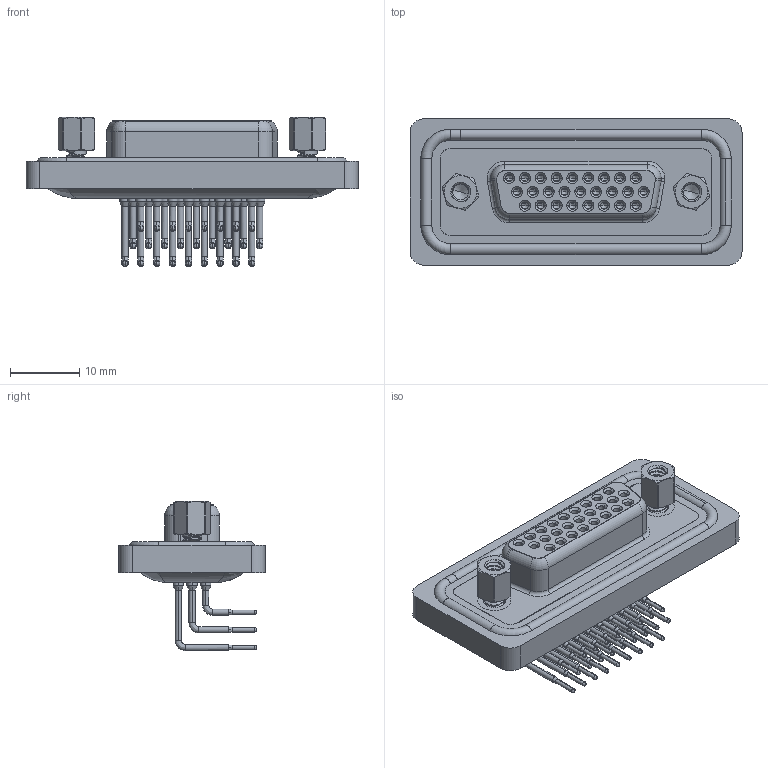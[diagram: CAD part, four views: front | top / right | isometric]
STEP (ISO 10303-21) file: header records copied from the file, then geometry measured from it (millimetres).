
FILE_DESCRIPTION (( 'STEP AP203' ), '1' );
FILE_NAME ('634-W26-662-012.STEP', '2024-04-12T19:19:04', ( '' ), ( '' ), 'SwSTEP 2.0', 'SolidWorks 2023', '' );
FILE_SCHEMA (( 'CONFIG_CONTROL_DESIGN' ));
Length unit declared in the file: millimetre
Products named in the file (9): 634-W26-662-012; 634W 4-40 Hex Standoff; 634W Contact Row 1; 634W Contact Row 2; 634W 4-40 Threaded Rivet; 634W Waterproof Housing_26 Contacts; 634W Housing_26 Contacts; 634W Contact Row 3; 634W Shell_26 Contacts
Assembly tree (33 placements, depth 2):
  634-W26-662-012
    634W Housing_26 Contacts
    634W Shell_26 Contacts
    634W Contact Row 1  x9
    634W Contact Row 2  x9
    634W Contact Row 3  x8
    634W 4-40 Threaded Rivet  x2
    634W Waterproof Housing_26 Contacts
    634W 4-40 Hex Standoff  x2
Bounding box: 47.89 x 21.1 x 21.52 mm (x, y, z)
Volume: 5559.2 mm3; surface area: 11557.5 mm2
Topology: 34 solids, 34 shells, 1853 faces, 4742 edges, 2994 vertices
Faces by surface type: cylinder 870, plane 491, cone 316, bspline 126, torus 50
Entity records: 30713 total; most frequent: CARTESIAN_POINT 8882, DIRECTION 4543, ORIENTED_EDGE 4014, EDGE_CURVE 2007, AXIS2_PLACEMENT_3D 1887, VERTEX_POINT 1288, EDGE_LOOP 1049, CIRCLE 1040
